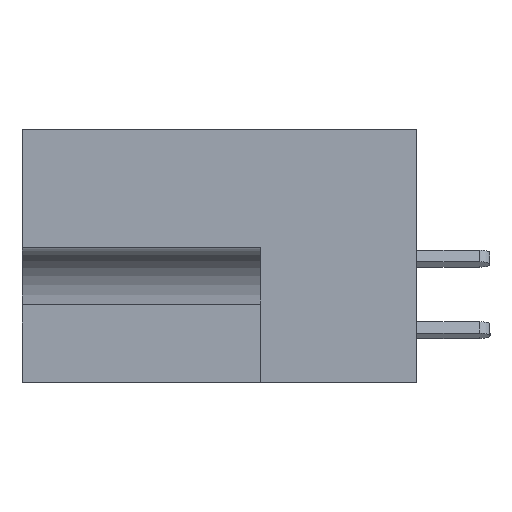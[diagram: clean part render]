
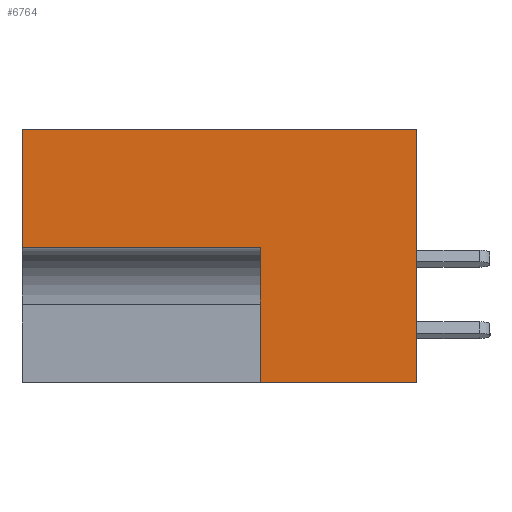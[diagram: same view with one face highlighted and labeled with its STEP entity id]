
A CAD part, left-side view. The second image highlights one B-rep face of the part: STEP entity #6764.
In plain terms, the highlighted planar face has unit normal (-1, 0, 0).
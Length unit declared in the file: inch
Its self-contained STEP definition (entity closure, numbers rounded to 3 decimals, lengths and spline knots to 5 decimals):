
#263 = FACE_OUTER_BOUND ( 'NONE', #3570, .T. ) ;
#561 = DIRECTION ( 'NONE',  ( 0., 0., 1. ) ) ;
#692 = CARTESIAN_POINT ( 'NONE',  ( 0., 0.453, -0.531 ) ) ;
#738 = PLANE ( 'NONE',  #4365 ) ;
#797 = CARTESIAN_POINT ( 'NONE',  ( 0., 0., 0. ) ) ;
#1020 = EDGE_CURVE ( 'NONE', #16985, #4492, #1921, .T. ) ;
#1384 = DIRECTION ( 'NONE',  ( 0., 1., 0. ) ) ;
#1743 = CARTESIAN_POINT ( 'NONE',  ( 0., 0., 0. ) ) ;
#1921 = LINE ( 'NONE', #8820, #5706 ) ;
#2397 = VERTEX_POINT ( 'NONE', #11352 ) ;
#2443 = CARTESIAN_POINT ( 'NONE',  ( 0., 0., -0.531 ) ) ;
#2745 = VECTOR ( 'NONE', #1384, 39.37008 ) ;
#3232 = DIRECTION ( 'NONE',  ( 0., -1., 0. ) ) ;
#3570 = EDGE_LOOP ( 'NONE', ( #16679, #11094, #12078, #9527, #13121, #17057 ) ) ;
#4365 = AXIS2_PLACEMENT_3D ( 'NONE', #9909, #10146, #7344 ) ;
#4492 = VERTEX_POINT ( 'NONE', #1743 ) ;
#5628 = VERTEX_POINT ( 'NONE', #10800 ) ;
#5706 = VECTOR ( 'NONE', #3232, 39.37008 ) ;
#5844 = VERTEX_POINT ( 'NONE', #2443 ) ;
#6764 = ADVANCED_FACE ( 'NONE', ( #263 ), #738, .F. ) ;
#6768 = CARTESIAN_POINT ( 'NONE',  ( 0., 0.328, -0.531 ) ) ;
#7344 = DIRECTION ( 'NONE',  ( 0., 0., -1. ) ) ;
#7403 = CARTESIAN_POINT ( 'NONE',  ( 0., 0.328, -0.248 ) ) ;
#7537 = DIRECTION ( 'NONE',  ( 0., -1., 0. ) ) ;
#7786 = CARTESIAN_POINT ( 'NONE',  ( 0., 0.328, -0.248 ) ) ;
#7957 = VECTOR ( 'NONE', #16752, 39.37008 ) ;
#8193 = EDGE_CURVE ( 'NONE', #5628, #16985, #8225, .T. ) ;
#8225 = LINE ( 'NONE', #8566, #15158 ) ;
#8271 = CARTESIAN_POINT ( 'NONE',  ( 0., 0.828, 0. ) ) ;
#8566 = CARTESIAN_POINT ( 'NONE',  ( 0., 0.828, 0. ) ) ;
#8820 = CARTESIAN_POINT ( 'NONE',  ( 0., 0.453, 0. ) ) ;
#8844 = EDGE_CURVE ( 'NONE', #2397, #10100, #11116, .T. ) ;
#9527 = ORIENTED_EDGE ( 'NONE', *, *, #11239, .T. ) ;
#9614 = LINE ( 'NONE', #797, #7957 ) ;
#9717 = EDGE_CURVE ( 'NONE', #5844, #4492, #9614, .T. ) ;
#9909 = CARTESIAN_POINT ( 'NONE',  ( 0., 0.453, 0. ) ) ;
#10100 = VERTEX_POINT ( 'NONE', #7403 ) ;
#10146 = DIRECTION ( 'NONE',  ( 1., 0., 0. ) ) ;
#10800 = CARTESIAN_POINT ( 'NONE',  ( 0., 0.828, -0.248 ) ) ;
#11030 = LINE ( 'NONE', #692, #16096 ) ;
#11094 = ORIENTED_EDGE ( 'NONE', *, *, #14459, .F. ) ;
#11116 = LINE ( 'NONE', #6768, #11562 ) ;
#11239 = EDGE_CURVE ( 'NONE', #2397, #5844, #11030, .T. ) ;
#11352 = CARTESIAN_POINT ( 'NONE',  ( 0., 0.328, -0.531 ) ) ;
#11562 = VECTOR ( 'NONE', #14917, 39.37008 ) ;
#12078 = ORIENTED_EDGE ( 'NONE', *, *, #8844, .F. ) ;
#13121 = ORIENTED_EDGE ( 'NONE', *, *, #9717, .T. ) ;
#14459 = EDGE_CURVE ( 'NONE', #10100, #5628, #16226, .T. ) ;
#14917 = DIRECTION ( 'NONE',  ( 0., 0., 1. ) ) ;
#15158 = VECTOR ( 'NONE', #561, 39.37008 ) ;
#16096 = VECTOR ( 'NONE', #7537, 39.37008 ) ;
#16226 = LINE ( 'NONE', #7786, #2745 ) ;
#16679 = ORIENTED_EDGE ( 'NONE', *, *, #8193, .F. ) ;
#16752 = DIRECTION ( 'NONE',  ( 0., 0., 1. ) ) ;
#16985 = VERTEX_POINT ( 'NONE', #8271 ) ;
#17057 = ORIENTED_EDGE ( 'NONE', *, *, #1020, .F. ) ;
